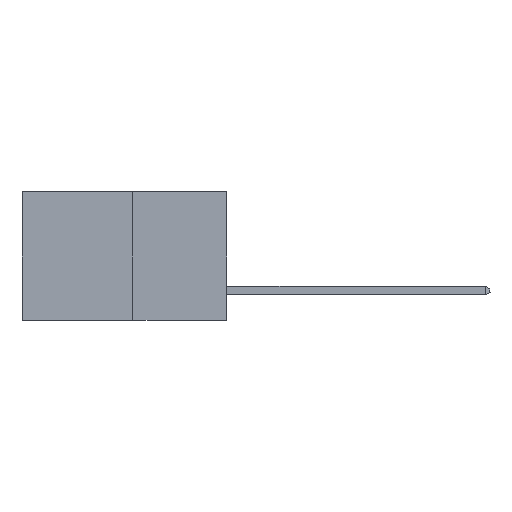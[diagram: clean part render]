
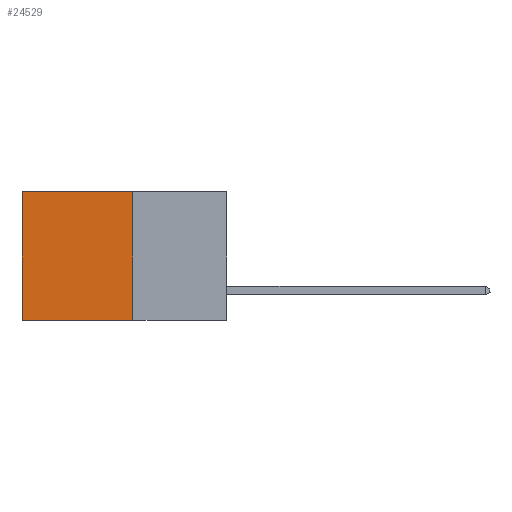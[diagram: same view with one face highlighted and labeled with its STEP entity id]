
A CAD part, left-side view. The second image highlights one B-rep face of the part: STEP entity #24529.
In plain terms, the highlighted planar face has unit normal (-1, 0, 0).
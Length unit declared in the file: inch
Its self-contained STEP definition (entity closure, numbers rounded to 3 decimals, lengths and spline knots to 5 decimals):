
#124 = DIRECTION ( 'NONE',  ( 0., 0., -1. ) ) ;
#370 = CARTESIAN_POINT ( 'NONE',  ( 0.277, 0.27, -0.37 ) ) ;
#832 = ORIENTED_EDGE ( 'NONE', *, *, #15982, .T. ) ;
#2229 = VECTOR ( 'NONE', #22940, 39.37008 ) ;
#2896 = LINE ( 'NONE', #12867, #2229 ) ;
#4050 = VECTOR ( 'NONE', #18386, 39.37008 ) ;
#4248 = EDGE_CURVE ( 'NONE', #16831, #16453, #18364, .T. ) ;
#4708 = CARTESIAN_POINT ( 'NONE',  ( 0.277, 0.59, -0.37 ) ) ;
#4790 = VERTEX_POINT ( 'NONE', #6312 ) ;
#4882 = CARTESIAN_POINT ( 'NONE',  ( 0.277, 0.27, -0.37 ) ) ;
#6010 = CARTESIAN_POINT ( 'NONE',  ( 0.277, 0.27, -0.37 ) ) ;
#6312 = CARTESIAN_POINT ( 'NONE',  ( 0.277, 0.59, 0. ) ) ;
#7617 = AXIS2_PLACEMENT_3D ( 'NONE', #6010, #20139, #8030 ) ;
#8030 = DIRECTION ( 'NONE',  ( 0., 0., -1. ) ) ;
#8062 = EDGE_LOOP ( 'NONE', ( #832, #20651, #12971, #8936 ) ) ;
#8710 = VECTOR ( 'NONE', #18491, 39.37008 ) ;
#8936 = ORIENTED_EDGE ( 'NONE', *, *, #15306, .T. ) ;
#12867 = CARTESIAN_POINT ( 'NONE',  ( 0.277, 0.59, -0.37 ) ) ;
#12971 = ORIENTED_EDGE ( 'NONE', *, *, #4248, .F. ) ;
#13778 = CARTESIAN_POINT ( 'NONE',  ( 0.277, 0.27, 0. ) ) ;
#15192 = FACE_OUTER_BOUND ( 'NONE', #8062, .T. ) ;
#15306 = EDGE_CURVE ( 'NONE', #16831, #4790, #24767, .T. ) ;
#15982 = EDGE_CURVE ( 'NONE', #4790, #17846, #2896, .T. ) ;
#16322 = CARTESIAN_POINT ( 'NONE',  ( 0.277, 0.27, -0.37 ) ) ;
#16423 = CARTESIAN_POINT ( 'NONE',  ( 0.277, 0.27, 0. ) ) ;
#16453 = VERTEX_POINT ( 'NONE', #370 ) ;
#16831 = VERTEX_POINT ( 'NONE', #13778 ) ;
#17846 = VERTEX_POINT ( 'NONE', #4708 ) ;
#18084 = PLANE ( 'NONE',  #7617 ) ;
#18364 = LINE ( 'NONE', #4882, #23118 ) ;
#18386 = DIRECTION ( 'NONE',  ( 0., 1., 0. ) ) ;
#18491 = DIRECTION ( 'NONE',  ( 0., 1., 0. ) ) ;
#20139 = DIRECTION ( 'NONE',  ( 1., 0., 0. ) ) ;
#20327 = EDGE_CURVE ( 'NONE', #16453, #17846, #25533, .T. ) ;
#20651 = ORIENTED_EDGE ( 'NONE', *, *, #20327, .F. ) ;
#22940 = DIRECTION ( 'NONE',  ( 0., 0., -1. ) ) ;
#23118 = VECTOR ( 'NONE', #124, 39.37008 ) ;
#24529 = ADVANCED_FACE ( 'NONE', ( #15192 ), #18084, .F. ) ;
#24767 = LINE ( 'NONE', #16423, #8710 ) ;
#25533 = LINE ( 'NONE', #16322, #4050 ) ;
